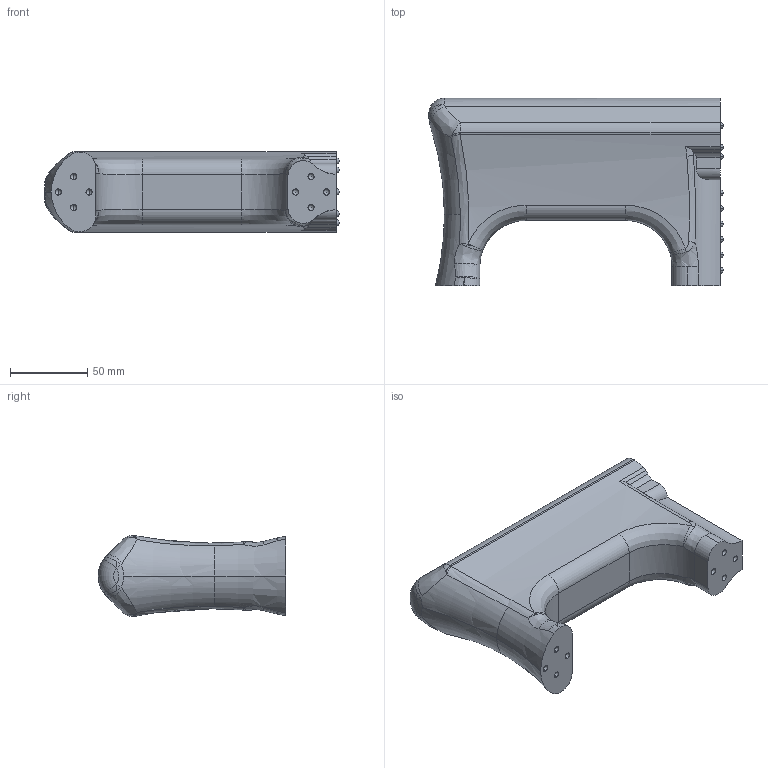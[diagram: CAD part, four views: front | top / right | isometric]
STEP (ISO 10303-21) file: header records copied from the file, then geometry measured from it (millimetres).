
FILE_DESCRIPTION (( 'STEP AP214' ), '1' );
FILE_NAME ('Stock_Rear1.STEP', '2013-10-07T07:00:07', ( 'elpi' ), ( '' ), 'SwSTEP 2.0', 'SolidWorks 2013', '' );
FILE_SCHEMA (( 'AUTOMOTIVE_DESIGN' ));
Length unit declared in the file: millimetre
Products named in the file (1): Stock_Rear1
Bounding box: 190.8 x 121.45 x 52.5 mm (x, y, z)
Volume: 623305.7 mm3; surface area: 67416.2 mm2
Topology: 1 solids, 1 shells, 133 faces, 370 edges, 221 vertices
Faces by surface type: sphere 48, bspline 33, cylinder 31, plane 14, torus 7
Entity records: 6296 total; most frequent: CARTESIAN_POINT 3516, ORIENTED_EDGE 588, DIRECTION 547, EDGE_CURVE 294, AXIS2_PLACEMENT_3D 247, VERTEX_POINT 183, EDGE_LOOP 153, CIRCLE 146
